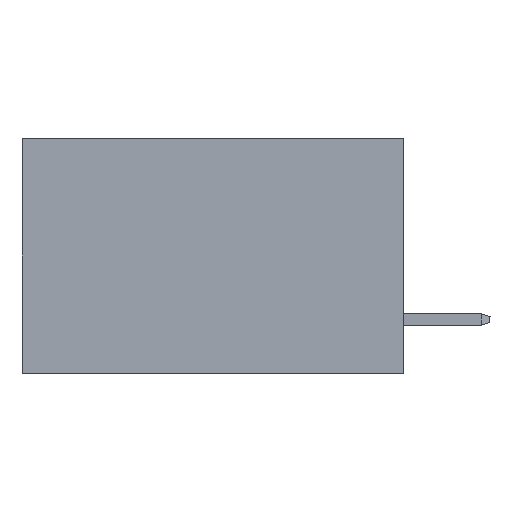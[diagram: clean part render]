
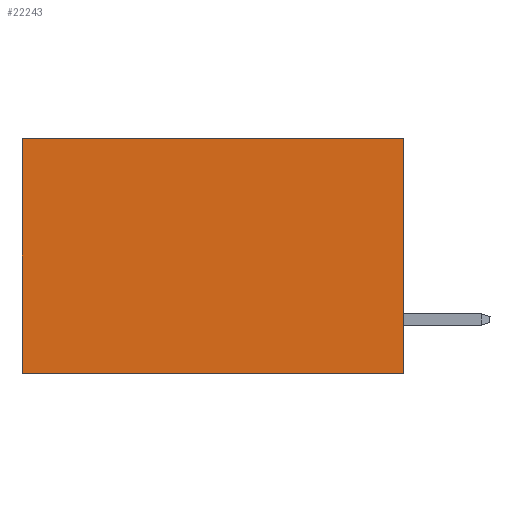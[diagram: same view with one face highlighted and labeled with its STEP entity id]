
A CAD part, left-side view. The second image highlights one B-rep face of the part: STEP entity #22243.
In plain terms, the highlighted planar face has unit normal (-1, 0, 0).
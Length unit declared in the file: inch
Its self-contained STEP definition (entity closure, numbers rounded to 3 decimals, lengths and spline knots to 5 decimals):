
#197 = FACE_OUTER_BOUND ( 'NONE', #744, .T. ) ;
#274 = CARTESIAN_POINT ( 'NONE',  ( 0.2875, 0.6, 0. ) ) ;
#744 = EDGE_LOOP ( 'NONE', ( #5420, #8455, #8308, #12567 ) ) ;
#2557 = LINE ( 'NONE', #274, #3724 ) ;
#2617 = EDGE_CURVE ( 'NONE', #15500, #16520, #2557, .T. ) ;
#3724 = VECTOR ( 'NONE', #5106, 39.37008 ) ;
#5028 = DIRECTION ( 'NONE',  ( 1., 0., 0. ) ) ;
#5106 = DIRECTION ( 'NONE',  ( 0., 0., -1. ) ) ;
#5420 = ORIENTED_EDGE ( 'NONE', *, *, #2617, .T. ) ;
#6153 = DIRECTION ( 'NONE',  ( 0., 1., 0. ) ) ;
#6919 = PLANE ( 'NONE',  #12876 ) ;
#7523 = CARTESIAN_POINT ( 'NONE',  ( 0.2875, 0., 0. ) ) ;
#8152 = VERTEX_POINT ( 'NONE', #14383 ) ;
#8308 = ORIENTED_EDGE ( 'NONE', *, *, #14968, .F. ) ;
#8455 = ORIENTED_EDGE ( 'NONE', *, *, #22914, .F. ) ;
#9033 = CARTESIAN_POINT ( 'NONE',  ( 0.2875, 0.6, 0. ) ) ;
#9540 = DIRECTION ( 'NONE',  ( 0., 1., 0. ) ) ;
#9811 = VECTOR ( 'NONE', #10533, 39.37008 ) ;
#10533 = DIRECTION ( 'NONE',  ( 0., 0., -1. ) ) ;
#10813 = LINE ( 'NONE', #15126, #9811 ) ;
#11143 = CARTESIAN_POINT ( 'NONE',  ( 0.2875, 0., 0. ) ) ;
#11229 = VECTOR ( 'NONE', #9540, 39.37008 ) ;
#12567 = ORIENTED_EDGE ( 'NONE', *, *, #16069, .T. ) ;
#12876 = AXIS2_PLACEMENT_3D ( 'NONE', #15974, #5028, #22550 ) ;
#14383 = CARTESIAN_POINT ( 'NONE',  ( 0.2875, 0., -0.37 ) ) ;
#14968 = EDGE_CURVE ( 'NONE', #25790, #8152, #10813, .T. ) ;
#15126 = CARTESIAN_POINT ( 'NONE',  ( 0.2875, 0., 0. ) ) ;
#15500 = VERTEX_POINT ( 'NONE', #9033 ) ;
#15974 = CARTESIAN_POINT ( 'NONE',  ( 0.2875, 0., 0. ) ) ;
#16069 = EDGE_CURVE ( 'NONE', #25790, #15500, #18441, .T. ) ;
#16520 = VERTEX_POINT ( 'NONE', #18552 ) ;
#18441 = LINE ( 'NONE', #7523, #11229 ) ;
#18552 = CARTESIAN_POINT ( 'NONE',  ( 0.2875, 0.6, -0.37 ) ) ;
#22243 = ADVANCED_FACE ( 'NONE', ( #197 ), #6919, .F. ) ;
#22494 = VECTOR ( 'NONE', #6153, 39.37008 ) ;
#22550 = DIRECTION ( 'NONE',  ( 0., 0., -1. ) ) ;
#22914 = EDGE_CURVE ( 'NONE', #8152, #16520, #23663, .T. ) ;
#23362 = CARTESIAN_POINT ( 'NONE',  ( 0.2875, 0., -0.37 ) ) ;
#23663 = LINE ( 'NONE', #23362, #22494 ) ;
#25790 = VERTEX_POINT ( 'NONE', #11143 ) ;
